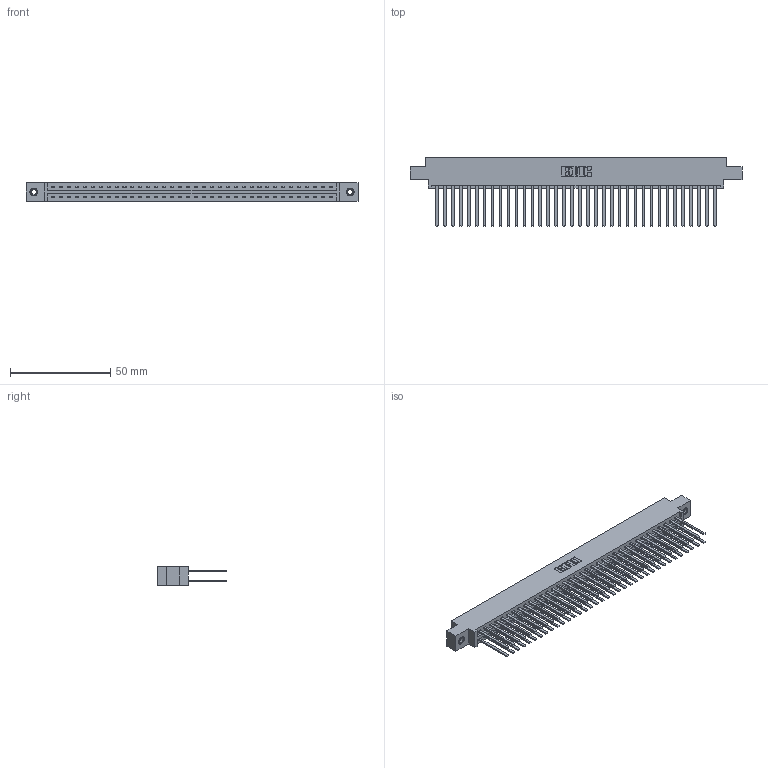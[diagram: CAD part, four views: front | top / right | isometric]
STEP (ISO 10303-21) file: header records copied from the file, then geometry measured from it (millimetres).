
FILE_DESCRIPTION (( 'STEP AP203' ), '1' );
FILE_NAME ('337-072-544-808.STEP', '2019-10-15T11:49:58', ( '' ), ( '' ), 'SwSTEP 2.0', 'SolidWorks 2016', '' );
FILE_SCHEMA (( 'CONFIG_CONTROL_DESIGN' ));
Length unit declared in the file: inch
Products named in the file (4): 337 Part_0.170 Offset - 0.156 Dia-TI; 337-072-544-808; 345-250-001_345-250-003-102; 345-292-001_345-293-144
Assembly tree (75 placements, depth 2):
  337-072-544-808
    337 Part_0.170 Offset - 0.156 Dia-TI
    345-292-001_345-293-144  x72
    345-250-001_345-250-003-102  x2
Bounding box: 165.66 x 34.3 x 9.4 mm (x, y, z)
Volume: 18263.9 mm3; surface area: 24017.9 mm2
Topology: 75 solids, 75 shells, 3634 faces, 10755 edges, 7066 vertices
Faces by surface type: plane 2554, cylinder 1064, cone 12, torus 4
Entity records: 29822 total; most frequent: CARTESIAN_POINT 5009, ORIENTED_EDGE 4938, DIRECTION 4299, EDGE_CURVE 2469, LINE 2325, VECTOR 2325, VERTEX_POINT 1640, AXIS2_PLACEMENT_3D 987
